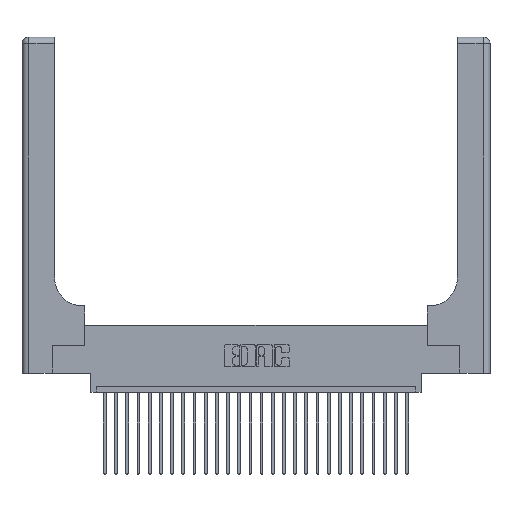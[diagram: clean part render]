
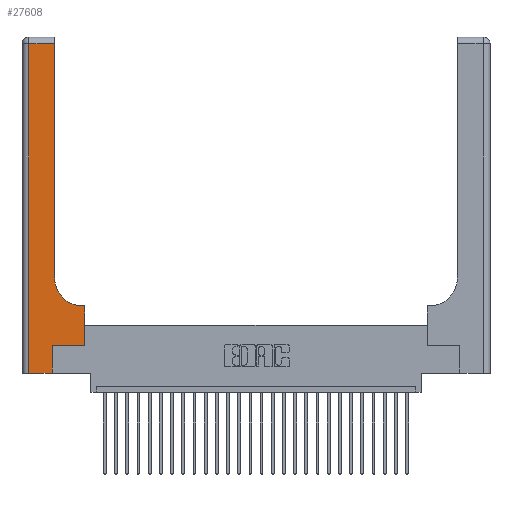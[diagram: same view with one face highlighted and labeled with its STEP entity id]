
A CAD part, top view. The second image highlights one B-rep face of the part: STEP entity #27608.
In plain terms, the highlighted planar face has unit normal (0, 0, 1).
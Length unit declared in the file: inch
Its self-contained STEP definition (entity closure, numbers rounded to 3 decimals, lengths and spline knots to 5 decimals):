
#167 = CARTESIAN_POINT ( 'NONE',  ( 0.5415, 0.6, 0.37 ) ) ;
#277 = DIRECTION ( 'NONE',  ( -1., 0., 0. ) ) ;
#479 = ORIENTED_EDGE ( 'NONE', *, *, #17600, .T. ) ;
#540 = FACE_OUTER_BOUND ( 'NONE', #7501, .T. ) ;
#1596 = LINE ( 'NONE', #24022, #24150 ) ;
#1734 = DIRECTION ( 'NONE',  ( 0., 0., -1. ) ) ;
#1914 = VECTOR ( 'NONE', #17568, 39.37008 ) ;
#2038 = VECTOR ( 'NONE', #8940, 39.37008 ) ;
#2195 = EDGE_CURVE ( 'NONE', #13234, #13409, #28260, .T. ) ;
#2522 = CARTESIAN_POINT ( 'NONE',  ( 0.2915, 0.6, 0.37 ) ) ;
#2609 = VECTOR ( 'NONE', #15875, 39.37008 ) ;
#3026 = EDGE_CURVE ( 'NONE', #12942, #13024, #7726, .T. ) ;
#4126 = CARTESIAN_POINT ( 'NONE',  ( 0., 3., 0.37 ) ) ;
#4902 = VERTEX_POINT ( 'NONE', #11654 ) ;
#5249 = CARTESIAN_POINT ( 'NONE',  ( 0.269, 0., 0.37 ) ) ;
#5354 = LINE ( 'NONE', #9296, #15586 ) ;
#5964 = ORIENTED_EDGE ( 'NONE', *, *, #2195, .T. ) ;
#7501 = EDGE_LOOP ( 'NONE', ( #18432, #5964, #479, #11781, #16551, #17241, #18654, #11135, #20813 ) ) ;
#7710 = CARTESIAN_POINT ( 'NONE',  ( 0.2915, 0.85, 0.37 ) ) ;
#7726 = LINE ( 'NONE', #25454, #15589 ) ;
#8389 = VECTOR ( 'NONE', #17354, 39.37008 ) ;
#8940 = DIRECTION ( 'NONE',  ( 1., 0., 0. ) ) ;
#9173 = CARTESIAN_POINT ( 'NONE',  ( 0.06, 2.94, 0.37 ) ) ;
#9296 = CARTESIAN_POINT ( 'NONE',  ( 0., 0., 0.37 ) ) ;
#9451 = EDGE_CURVE ( 'NONE', #12906, #12942, #5354, .T. ) ;
#9964 = CARTESIAN_POINT ( 'NONE',  ( 0.5585, 0.6, 0.37 ) ) ;
#9995 = EDGE_CURVE ( 'NONE', #21027, #26174, #10071, .T. ) ;
#10071 = CIRCLE ( 'NONE', #14295, 0.25 ) ;
#10575 = PLANE ( 'NONE',  #24511 ) ;
#11135 = ORIENTED_EDGE ( 'NONE', *, *, #19632, .T. ) ;
#11229 = CARTESIAN_POINT ( 'NONE',  ( 0.5415, 0.85, 0.37 ) ) ;
#11654 = CARTESIAN_POINT ( 'NONE',  ( 0.5585, 0.25, 0.37 ) ) ;
#11781 = ORIENTED_EDGE ( 'NONE', *, *, #9451, .T. ) ;
#12115 = LINE ( 'NONE', #23936, #8389 ) ;
#12645 = CARTESIAN_POINT ( 'NONE',  ( 0.2915, 2.94, 0.37 ) ) ;
#12664 = VERTEX_POINT ( 'NONE', #9964 ) ;
#12701 = LINE ( 'NONE', #2522, #23332 ) ;
#12906 = VERTEX_POINT ( 'NONE', #19586 ) ;
#12942 = VERTEX_POINT ( 'NONE', #5249 ) ;
#13024 = VERTEX_POINT ( 'NONE', #14809 ) ;
#13234 = VERTEX_POINT ( 'NONE', #12645 ) ;
#13322 = CARTESIAN_POINT ( 'NONE',  ( 0.269, 0.25, 0.37 ) ) ;
#13409 = VERTEX_POINT ( 'NONE', #9173 ) ;
#13427 = DIRECTION ( 'NONE',  ( 1., 0., 0. ) ) ;
#13572 = LINE ( 'NONE', #13322, #2038 ) ;
#14295 = AXIS2_PLACEMENT_3D ( 'NONE', #11229, #19699, #13427 ) ;
#14809 = CARTESIAN_POINT ( 'NONE',  ( 0.269, 0.25, 0.37 ) ) ;
#15586 = VECTOR ( 'NONE', #18149, 39.37008 ) ;
#15589 = VECTOR ( 'NONE', #25252, 39.37008 ) ;
#15619 = CARTESIAN_POINT ( 'NONE',  ( 0.2915, 3., 0.37 ) ) ;
#15875 = DIRECTION ( 'NONE',  ( -1., 0., 0. ) ) ;
#15928 = EDGE_CURVE ( 'NONE', #13024, #4902, #13572, .T. ) ;
#16551 = ORIENTED_EDGE ( 'NONE', *, *, #3026, .T. ) ;
#17241 = ORIENTED_EDGE ( 'NONE', *, *, #15928, .T. ) ;
#17354 = DIRECTION ( 'NONE',  ( 0., -1., 0. ) ) ;
#17568 = DIRECTION ( 'NONE',  ( 0., 1., 0. ) ) ;
#17600 = EDGE_CURVE ( 'NONE', #13409, #12906, #12115, .T. ) ;
#17760 = EDGE_CURVE ( 'NONE', #4902, #12664, #1596, .T. ) ;
#18149 = DIRECTION ( 'NONE',  ( 1., 0., 0. ) ) ;
#18432 = ORIENTED_EDGE ( 'NONE', *, *, #28200, .T. ) ;
#18654 = ORIENTED_EDGE ( 'NONE', *, *, #17760, .T. ) ;
#19586 = CARTESIAN_POINT ( 'NONE',  ( 0.06, 0., 0.37 ) ) ;
#19632 = EDGE_CURVE ( 'NONE', #12664, #21027, #12701, .T. ) ;
#19699 = DIRECTION ( 'NONE',  ( 0., 0., -1. ) ) ;
#20172 = DIRECTION ( 'NONE',  ( 0., 1., 0. ) ) ;
#20813 = ORIENTED_EDGE ( 'NONE', *, *, #9995, .T. ) ;
#21027 = VERTEX_POINT ( 'NONE', #167 ) ;
#21043 = LINE ( 'NONE', #15619, #1914 ) ;
#23332 = VECTOR ( 'NONE', #26708, 39.37008 ) ;
#23936 = CARTESIAN_POINT ( 'NONE',  ( 0.06, 3., 0.37 ) ) ;
#24022 = CARTESIAN_POINT ( 'NONE',  ( 0.5585, 0.25, 0.37 ) ) ;
#24125 = CARTESIAN_POINT ( 'NONE',  ( 0., 2.94, 0.37 ) ) ;
#24150 = VECTOR ( 'NONE', #20172, 39.37008 ) ;
#24511 = AXIS2_PLACEMENT_3D ( 'NONE', #4126, #1734, #277 ) ;
#25252 = DIRECTION ( 'NONE',  ( 0., 1., 0. ) ) ;
#25454 = CARTESIAN_POINT ( 'NONE',  ( 0.269, 0., 0.37 ) ) ;
#26174 = VERTEX_POINT ( 'NONE', #7710 ) ;
#26708 = DIRECTION ( 'NONE',  ( -1., 0., 0. ) ) ;
#27608 = ADVANCED_FACE ( 'NONE', ( #540 ), #10575, .F. ) ;
#28200 = EDGE_CURVE ( 'NONE', #26174, #13234, #21043, .T. ) ;
#28260 = LINE ( 'NONE', #24125, #2609 ) ;
